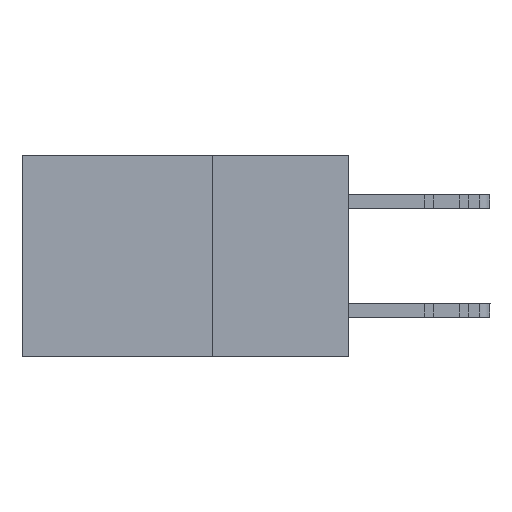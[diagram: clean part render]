
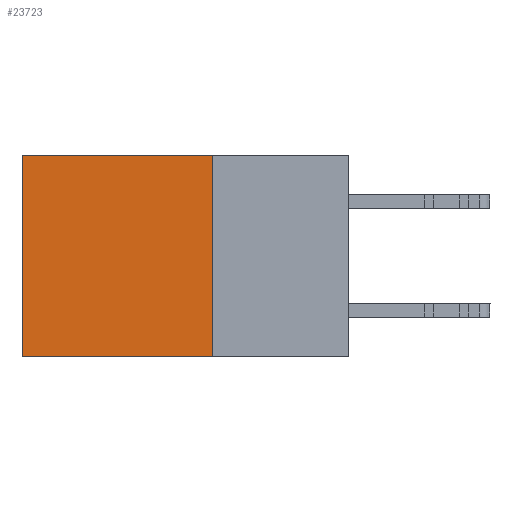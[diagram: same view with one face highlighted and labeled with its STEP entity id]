
A CAD part, left-side view. The second image highlights one B-rep face of the part: STEP entity #23723.
In plain terms, the highlighted planar face has unit normal (-1, 0, 0).
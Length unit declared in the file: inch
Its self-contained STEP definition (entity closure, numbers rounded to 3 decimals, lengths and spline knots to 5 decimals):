
#535 = ORIENTED_EDGE ( 'NONE', *, *, #24443, .F. ) ;
#1100 = EDGE_LOOP ( 'NONE', ( #27638, #13427, #535, #11284 ) ) ;
#3422 = CARTESIAN_POINT ( 'NONE',  ( 0.298, 0.6, 0. ) ) ;
#4418 = CARTESIAN_POINT ( 'NONE',  ( 0.298, 0.25, -0.37 ) ) ;
#5335 = EDGE_CURVE ( 'NONE', #6460, #14091, #19471, .T. ) ;
#6460 = VERTEX_POINT ( 'NONE', #10638 ) ;
#6467 = CARTESIAN_POINT ( 'NONE',  ( 0.298, 0.25, 0. ) ) ;
#7284 = VECTOR ( 'NONE', #11819, 39.37008 ) ;
#7991 = VECTOR ( 'NONE', #14285, 39.37008 ) ;
#9113 = CARTESIAN_POINT ( 'NONE',  ( 0.298, 0.25, 0. ) ) ;
#9132 = DIRECTION ( 'NONE',  ( 0., 1., 0. ) ) ;
#9411 = DIRECTION ( 'NONE',  ( 1., 0., 0. ) ) ;
#10638 = CARTESIAN_POINT ( 'NONE',  ( 0.298, 0.25, -0.37 ) ) ;
#10778 = CARTESIAN_POINT ( 'NONE',  ( 0.298, 0.6, -0.37 ) ) ;
#11284 = ORIENTED_EDGE ( 'NONE', *, *, #27729, .T. ) ;
#11310 = LINE ( 'NONE', #3422, #7991 ) ;
#11457 = LINE ( 'NONE', #21064, #24676 ) ;
#11819 = DIRECTION ( 'NONE',  ( 0., 0., -1. ) ) ;
#12835 = EDGE_CURVE ( 'NONE', #22681, #14091, #11310, .T. ) ;
#13427 = ORIENTED_EDGE ( 'NONE', *, *, #5335, .F. ) ;
#13693 = VERTEX_POINT ( 'NONE', #6467 ) ;
#14091 = VERTEX_POINT ( 'NONE', #10778 ) ;
#14285 = DIRECTION ( 'NONE',  ( 0., 0., -1. ) ) ;
#16000 = VECTOR ( 'NONE', #19584, 39.37008 ) ;
#16009 = PLANE ( 'NONE',  #20057 ) ;
#19471 = LINE ( 'NONE', #4418, #16000 ) ;
#19584 = DIRECTION ( 'NONE',  ( 0., 1., 0. ) ) ;
#20057 = AXIS2_PLACEMENT_3D ( 'NONE', #9113, #9411, #22107 ) ;
#21064 = CARTESIAN_POINT ( 'NONE',  ( 0.298, 0.25, 0. ) ) ;
#21139 = CARTESIAN_POINT ( 'NONE',  ( 0.298, 0.6, 0. ) ) ;
#22107 = DIRECTION ( 'NONE',  ( 0., 0., -1. ) ) ;
#22681 = VERTEX_POINT ( 'NONE', #21139 ) ;
#23723 = ADVANCED_FACE ( 'NONE', ( #26925 ), #16009, .F. ) ;
#24443 = EDGE_CURVE ( 'NONE', #13693, #6460, #27885, .T. ) ;
#24609 = CARTESIAN_POINT ( 'NONE',  ( 0.298, 0.25, 0. ) ) ;
#24676 = VECTOR ( 'NONE', #9132, 39.37008 ) ;
#26925 = FACE_OUTER_BOUND ( 'NONE', #1100, .T. ) ;
#27638 = ORIENTED_EDGE ( 'NONE', *, *, #12835, .T. ) ;
#27729 = EDGE_CURVE ( 'NONE', #13693, #22681, #11457, .T. ) ;
#27885 = LINE ( 'NONE', #24609, #7284 ) ;
